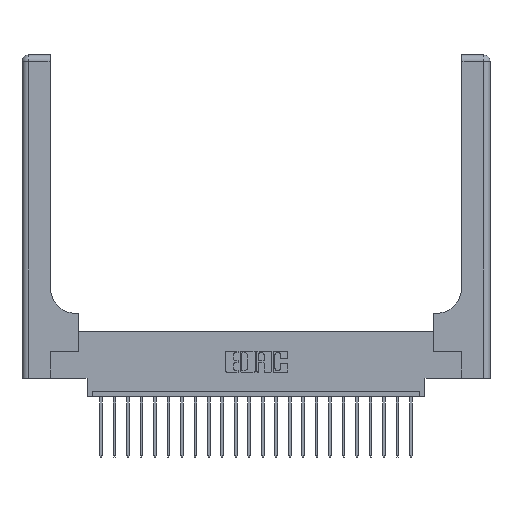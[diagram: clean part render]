
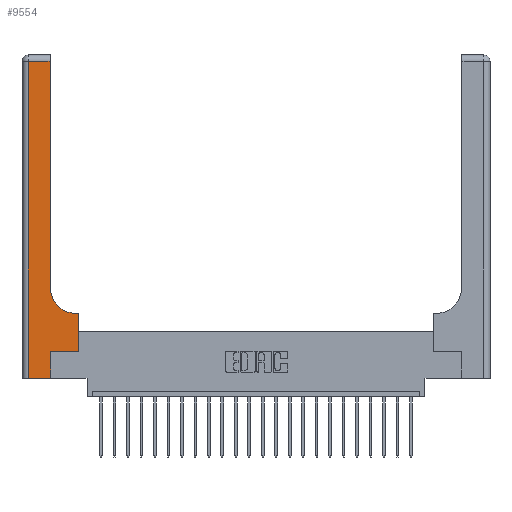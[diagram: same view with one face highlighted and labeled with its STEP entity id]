
A CAD part, top view. The second image highlights one B-rep face of the part: STEP entity #9554.
In plain terms, the highlighted planar face has unit normal (0, 0, 1).
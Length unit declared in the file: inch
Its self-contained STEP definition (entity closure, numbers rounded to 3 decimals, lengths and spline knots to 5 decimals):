
#522 = LINE ( 'NONE', #16190, #7429 ) ;
#533 = AXIS2_PLACEMENT_3D ( 'NONE', #1859, #17635, #19366 ) ;
#952 = DIRECTION ( 'NONE',  ( 1., 0., 0. ) ) ;
#1098 = ORIENTED_EDGE ( 'NONE', *, *, #7750, .T. ) ;
#1111 = DIRECTION ( 'NONE',  ( 0., 1., 0. ) ) ;
#1122 = CIRCLE ( 'NONE', #533, 0.25 ) ;
#1159 = EDGE_CURVE ( 'NONE', #20086, #22069, #522, .T. ) ;
#1605 = VERTEX_POINT ( 'NONE', #12029 ) ;
#1720 = VERTEX_POINT ( 'NONE', #9203 ) ;
#1859 = CARTESIAN_POINT ( 'NONE',  ( 0.51, 0.85, 0.37 ) ) ;
#1891 = VECTOR ( 'NONE', #952, 39.37008 ) ;
#2020 = EDGE_CURVE ( 'NONE', #8331, #20086, #16838, .T. ) ;
#2513 = PLANE ( 'NONE',  #19899 ) ;
#2721 = VECTOR ( 'NONE', #14065, 39.37008 ) ;
#2964 = CARTESIAN_POINT ( 'NONE',  ( 0.528, 0.25, 0.37 ) ) ;
#4010 = VECTOR ( 'NONE', #12158, 39.37008 ) ;
#4633 = ORIENTED_EDGE ( 'NONE', *, *, #15369, .T. ) ;
#4789 = CARTESIAN_POINT ( 'NONE',  ( 0.26, 0.6, 0.37 ) ) ;
#5498 = CARTESIAN_POINT ( 'NONE',  ( 0.265, 0., 0.37 ) ) ;
#5713 = DIRECTION ( 'NONE',  ( 0., 1., 0. ) ) ;
#5984 = ORIENTED_EDGE ( 'NONE', *, *, #12984, .T. ) ;
#6481 = DIRECTION ( 'NONE',  ( 1., 0., 0. ) ) ;
#6534 = EDGE_CURVE ( 'NONE', #20301, #13446, #12210, .T. ) ;
#6972 = FACE_OUTER_BOUND ( 'NONE', #8383, .T. ) ;
#7226 = CARTESIAN_POINT ( 'NONE',  ( 0.06, 3., 0.37 ) ) ;
#7395 = LINE ( 'NONE', #7226, #2721 ) ;
#7429 = VECTOR ( 'NONE', #5713, 39.37008 ) ;
#7703 = CARTESIAN_POINT ( 'NONE',  ( 0.51, 0.6, 0.37 ) ) ;
#7750 = EDGE_CURVE ( 'NONE', #1605, #19313, #22546, .T. ) ;
#7909 = CARTESIAN_POINT ( 'NONE',  ( 0., 0., 0.37 ) ) ;
#8331 = VERTEX_POINT ( 'NONE', #10034 ) ;
#8383 = EDGE_LOOP ( 'NONE', ( #12522, #12006, #11176, #15897, #17030, #5984, #4633, #1098, #16217 ) ) ;
#8544 = EDGE_CURVE ( 'NONE', #1720, #8331, #7395, .T. ) ;
#9030 = LINE ( 'NONE', #9337, #19411 ) ;
#9203 = CARTESIAN_POINT ( 'NONE',  ( 0.06, 2.94, 0.37 ) ) ;
#9337 = CARTESIAN_POINT ( 'NONE',  ( 0., 2.94, 0.37 ) ) ;
#9554 = ADVANCED_FACE ( 'NONE', ( #6972 ), #2513, .F. ) ;
#10034 = CARTESIAN_POINT ( 'NONE',  ( 0.06, 0., 0.37 ) ) ;
#10250 = VECTOR ( 'NONE', #17001, 39.37008 ) ;
#11152 = DIRECTION ( 'NONE',  ( -1., 0., 0. ) ) ;
#11176 = ORIENTED_EDGE ( 'NONE', *, *, #8544, .T. ) ;
#11320 = VECTOR ( 'NONE', #6481, 39.37008 ) ;
#11759 = CARTESIAN_POINT ( 'NONE',  ( 0.528, 0.25, 0.37 ) ) ;
#12006 = ORIENTED_EDGE ( 'NONE', *, *, #12373, .T. ) ;
#12029 = CARTESIAN_POINT ( 'NONE',  ( 0.528, 0.6, 0.37 ) ) ;
#12158 = DIRECTION ( 'NONE',  ( 0., 1., 0. ) ) ;
#12210 = LINE ( 'NONE', #22634, #4010 ) ;
#12373 = EDGE_CURVE ( 'NONE', #13446, #1720, #9030, .T. ) ;
#12522 = ORIENTED_EDGE ( 'NONE', *, *, #6534, .T. ) ;
#12984 = EDGE_CURVE ( 'NONE', #22069, #21012, #18582, .T. ) ;
#13012 = DIRECTION ( 'NONE',  ( -1., 0., 0. ) ) ;
#13446 = VERTEX_POINT ( 'NONE', #19627 ) ;
#14065 = DIRECTION ( 'NONE',  ( 0., -1., 0. ) ) ;
#14747 = CARTESIAN_POINT ( 'NONE',  ( 0., 3., 0.37 ) ) ;
#14890 = CARTESIAN_POINT ( 'NONE',  ( 0.26, 0.85, 0.37 ) ) ;
#15115 = CARTESIAN_POINT ( 'NONE',  ( 0.265, 0.25, 0.37 ) ) ;
#15369 = EDGE_CURVE ( 'NONE', #21012, #1605, #20602, .T. ) ;
#15897 = ORIENTED_EDGE ( 'NONE', *, *, #2020, .T. ) ;
#16190 = CARTESIAN_POINT ( 'NONE',  ( 0.265, 0., 0.37 ) ) ;
#16217 = ORIENTED_EDGE ( 'NONE', *, *, #17712, .T. ) ;
#16249 = VECTOR ( 'NONE', #1111, 39.37008 ) ;
#16838 = LINE ( 'NONE', #7909, #11320 ) ;
#17001 = DIRECTION ( 'NONE',  ( -1., 0., 0. ) ) ;
#17030 = ORIENTED_EDGE ( 'NONE', *, *, #1159, .T. ) ;
#17635 = DIRECTION ( 'NONE',  ( 0., 0., -1. ) ) ;
#17712 = EDGE_CURVE ( 'NONE', #19313, #20301, #1122, .T. ) ;
#18582 = LINE ( 'NONE', #15115, #1891 ) ;
#19313 = VERTEX_POINT ( 'NONE', #7703 ) ;
#19366 = DIRECTION ( 'NONE',  ( 1., 0., 0. ) ) ;
#19411 = VECTOR ( 'NONE', #13012, 39.37008 ) ;
#19627 = CARTESIAN_POINT ( 'NONE',  ( 0.26, 2.94, 0.37 ) ) ;
#19899 = AXIS2_PLACEMENT_3D ( 'NONE', #14747, #21691, #11152 ) ;
#20086 = VERTEX_POINT ( 'NONE', #5498 ) ;
#20301 = VERTEX_POINT ( 'NONE', #14890 ) ;
#20437 = CARTESIAN_POINT ( 'NONE',  ( 0.265, 0.25, 0.37 ) ) ;
#20602 = LINE ( 'NONE', #2964, #16249 ) ;
#21012 = VERTEX_POINT ( 'NONE', #11759 ) ;
#21691 = DIRECTION ( 'NONE',  ( 0., 0., -1. ) ) ;
#22069 = VERTEX_POINT ( 'NONE', #20437 ) ;
#22546 = LINE ( 'NONE', #4789, #10250 ) ;
#22634 = CARTESIAN_POINT ( 'NONE',  ( 0.26, 3., 0.37 ) ) ;
